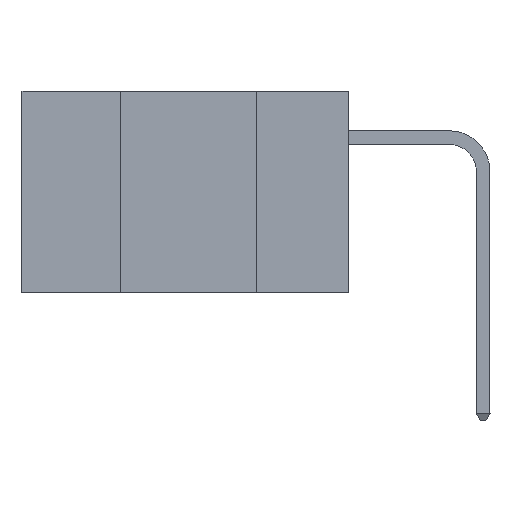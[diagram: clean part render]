
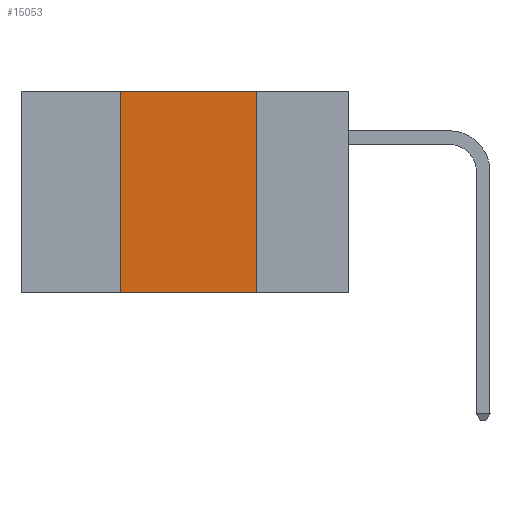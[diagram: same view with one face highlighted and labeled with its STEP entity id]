
A CAD part, left-side view. The second image highlights one B-rep face of the part: STEP entity #15053.
In plain terms, the highlighted planar face has unit normal (-1, 0, 0).
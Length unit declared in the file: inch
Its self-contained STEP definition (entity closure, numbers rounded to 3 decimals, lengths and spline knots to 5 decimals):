
#3640 = CARTESIAN_POINT ( 'NONE',  ( 0., 0.17, 0. ) ) ;
#5016 = DIRECTION ( 'NONE',  ( 0., -1., 0. ) ) ;
#6777 = EDGE_LOOP ( 'NONE', ( #12756, #26475, #15952, #9828 ) ) ;
#7365 = CARTESIAN_POINT ( 'NONE',  ( 0., 0.17, 0. ) ) ;
#7501 = CARTESIAN_POINT ( 'NONE',  ( 0., 0.42, 0. ) ) ;
#7926 = DIRECTION ( 'NONE',  ( 0., 0., -1. ) ) ;
#8827 = EDGE_CURVE ( 'NONE', #25197, #25458, #8926, .T. ) ;
#8876 = VECTOR ( 'NONE', #5016, 39.37008 ) ;
#8926 = LINE ( 'NONE', #23578, #17978 ) ;
#9237 = CARTESIAN_POINT ( 'NONE',  ( 0., 0.17, -0.37 ) ) ;
#9828 = ORIENTED_EDGE ( 'NONE', *, *, #10793, .T. ) ;
#10113 = LINE ( 'NONE', #19103, #11447 ) ;
#10518 = DIRECTION ( 'NONE',  ( 0., -1., 0. ) ) ;
#10543 = CARTESIAN_POINT ( 'NONE',  ( 0., 0.42, -0.37 ) ) ;
#10793 = EDGE_CURVE ( 'NONE', #25197, #14320, #10113, .T. ) ;
#11084 = VECTOR ( 'NONE', #7926, 39.37008 ) ;
#11447 = VECTOR ( 'NONE', #10518, 39.37008 ) ;
#12756 = ORIENTED_EDGE ( 'NONE', *, *, #18577, .F. ) ;
#14014 = LINE ( 'NONE', #3640, #11084 ) ;
#14320 = VERTEX_POINT ( 'NONE', #9237 ) ;
#15053 = ADVANCED_FACE ( 'NONE', ( #21066 ), #18593, .F. ) ;
#15277 = CARTESIAN_POINT ( 'NONE',  ( 0., 0.6, 0. ) ) ;
#15952 = ORIENTED_EDGE ( 'NONE', *, *, #8827, .F. ) ;
#17373 = DIRECTION ( 'NONE',  ( 0., 0., 1. ) ) ;
#17751 = DIRECTION ( 'NONE',  ( 0., 0., -1. ) ) ;
#17978 = VECTOR ( 'NONE', #17373, 39.37008 ) ;
#18175 = AXIS2_PLACEMENT_3D ( 'NONE', #15277, #25763, #17751 ) ;
#18577 = EDGE_CURVE ( 'NONE', #25330, #14320, #14014, .T. ) ;
#18593 = PLANE ( 'NONE',  #18175 ) ;
#18853 = EDGE_CURVE ( 'NONE', #25458, #25330, #23945, .T. ) ;
#19103 = CARTESIAN_POINT ( 'NONE',  ( 0., 0.6, -0.37 ) ) ;
#21066 = FACE_OUTER_BOUND ( 'NONE', #6777, .T. ) ;
#21730 = CARTESIAN_POINT ( 'NONE',  ( 0., 0.6, 0. ) ) ;
#23578 = CARTESIAN_POINT ( 'NONE',  ( 0., 0.42, 0. ) ) ;
#23945 = LINE ( 'NONE', #21730, #8876 ) ;
#25197 = VERTEX_POINT ( 'NONE', #10543 ) ;
#25330 = VERTEX_POINT ( 'NONE', #7365 ) ;
#25458 = VERTEX_POINT ( 'NONE', #7501 ) ;
#25763 = DIRECTION ( 'NONE',  ( 1., 0., 0. ) ) ;
#26475 = ORIENTED_EDGE ( 'NONE', *, *, #18853, .F. ) ;
